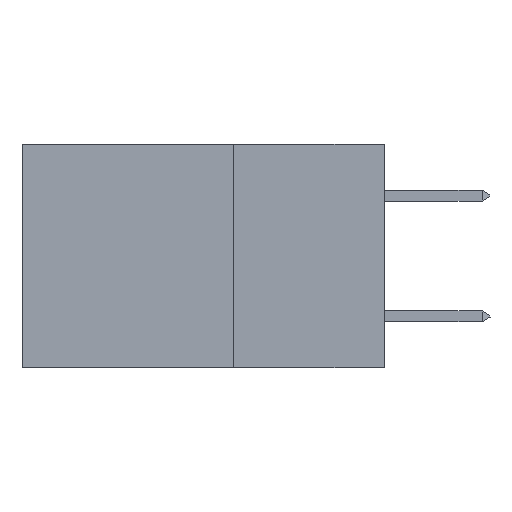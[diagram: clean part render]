
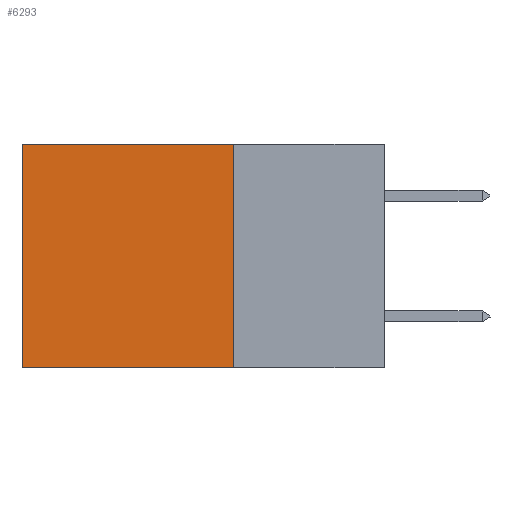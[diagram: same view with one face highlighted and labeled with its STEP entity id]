
A CAD part, left-side view. The second image highlights one B-rep face of the part: STEP entity #6293.
In plain terms, the highlighted planar face has unit normal (-1, 0, 0).
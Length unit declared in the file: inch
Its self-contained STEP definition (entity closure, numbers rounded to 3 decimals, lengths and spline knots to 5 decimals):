
#13 = EDGE_CURVE ( 'NONE', #3866, #2196, #8510, .T. ) ;
#305 = DIRECTION ( 'NONE',  ( 0., 1., 0. ) ) ;
#664 = FACE_OUTER_BOUND ( 'NONE', #2894, .T. ) ;
#1383 = CARTESIAN_POINT ( 'NONE',  ( 0.2875, 0.6, 0. ) ) ;
#2196 = VERTEX_POINT ( 'NONE', #1383 ) ;
#2849 = DIRECTION ( 'NONE',  ( 1., 0., 0. ) ) ;
#2860 = ORIENTED_EDGE ( 'NONE', *, *, #13, .T. ) ;
#2894 = EDGE_LOOP ( 'NONE', ( #6585, #7939, #7635, #2860 ) ) ;
#3866 = VERTEX_POINT ( 'NONE', #4469 ) ;
#4362 = CARTESIAN_POINT ( 'NONE',  ( 0.2875, 0.25, 0. ) ) ;
#4469 = CARTESIAN_POINT ( 'NONE',  ( 0.2875, 0.25, 0. ) ) ;
#4506 = EDGE_CURVE ( 'NONE', #3866, #8267, #5270, .T. ) ;
#4773 = VECTOR ( 'NONE', #9532, 39.37008 ) ;
#4820 = CARTESIAN_POINT ( 'NONE',  ( 0.2875, 0.25, -0.37 ) ) ;
#5233 = DIRECTION ( 'NONE',  ( 0., 0., -1. ) ) ;
#5270 = LINE ( 'NONE', #8164, #6530 ) ;
#5276 = VECTOR ( 'NONE', #8231, 39.37008 ) ;
#5518 = EDGE_CURVE ( 'NONE', #2196, #8795, #8954, .T. ) ;
#5722 = CARTESIAN_POINT ( 'NONE',  ( 0.2875, 0.6, -0.37 ) ) ;
#5798 = CARTESIAN_POINT ( 'NONE',  ( 0.2875, 0.25, 0. ) ) ;
#6096 = LINE ( 'NONE', #4820, #7959 ) ;
#6293 = ADVANCED_FACE ( 'NONE', ( #664 ), #7319, .F. ) ;
#6530 = VECTOR ( 'NONE', #5233, 39.37008 ) ;
#6585 = ORIENTED_EDGE ( 'NONE', *, *, #5518, .T. ) ;
#7319 = PLANE ( 'NONE',  #7511 ) ;
#7511 = AXIS2_PLACEMENT_3D ( 'NONE', #4362, #2849, #9547 ) ;
#7635 = ORIENTED_EDGE ( 'NONE', *, *, #4506, .F. ) ;
#7852 = CARTESIAN_POINT ( 'NONE',  ( 0.2875, 0.6, 0. ) ) ;
#7939 = ORIENTED_EDGE ( 'NONE', *, *, #9476, .F. ) ;
#7959 = VECTOR ( 'NONE', #305, 39.37008 ) ;
#8164 = CARTESIAN_POINT ( 'NONE',  ( 0.2875, 0.25, 0. ) ) ;
#8231 = DIRECTION ( 'NONE',  ( 0., 1., 0. ) ) ;
#8267 = VERTEX_POINT ( 'NONE', #8274 ) ;
#8274 = CARTESIAN_POINT ( 'NONE',  ( 0.2875, 0.25, -0.37 ) ) ;
#8510 = LINE ( 'NONE', #5798, #5276 ) ;
#8795 = VERTEX_POINT ( 'NONE', #5722 ) ;
#8954 = LINE ( 'NONE', #7852, #4773 ) ;
#9476 = EDGE_CURVE ( 'NONE', #8267, #8795, #6096, .T. ) ;
#9532 = DIRECTION ( 'NONE',  ( 0., 0., -1. ) ) ;
#9547 = DIRECTION ( 'NONE',  ( 0., 0., -1. ) ) ;
